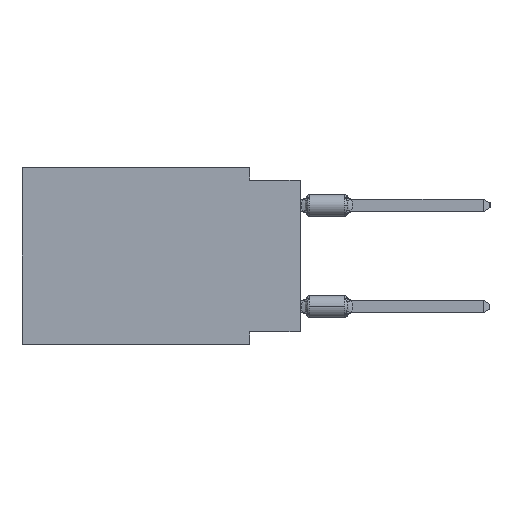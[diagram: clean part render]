
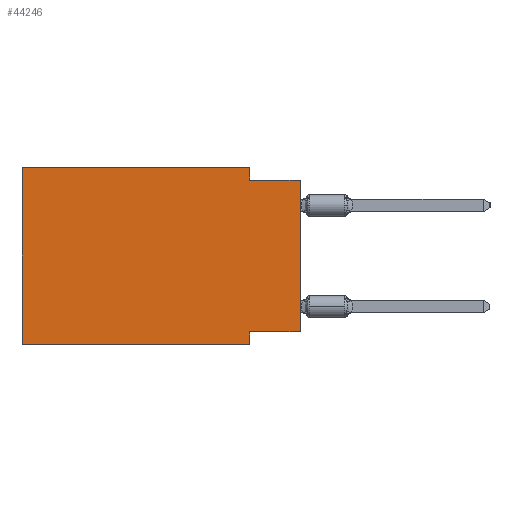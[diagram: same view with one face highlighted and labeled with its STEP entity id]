
A CAD part, left-side view. The second image highlights one B-rep face of the part: STEP entity #44246.
In plain terms, the highlighted planar face has unit normal (-1, 0, 0).
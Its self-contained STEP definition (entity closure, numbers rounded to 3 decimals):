
#1835 = ORIENTED_EDGE ( 'NONE', *, *, #51182, .T. ) ;
#3428 = CARTESIAN_POINT ( 'NONE',  ( 0., 13.97, -8.89 ) ) ;
#3501 = CARTESIAN_POINT ( 'NONE',  ( 0., 0., 0. ) ) ;
#4410 = EDGE_LOOP ( 'NONE', ( #1835, #31331, #40558, #20042, #10663, #21115, #50394, #46017 ) ) ;
#5445 = CARTESIAN_POINT ( 'NONE',  ( 0., 2.54, -8.89 ) ) ;
#5760 = LINE ( 'NONE', #50559, #7010 ) ;
#6490 = LINE ( 'NONE', #42623, #39428 ) ;
#6607 = CARTESIAN_POINT ( 'NONE',  ( 0., 0., -0.635 ) ) ;
#7010 = VECTOR ( 'NONE', #9966, 1000. ) ;
#7203 = EDGE_CURVE ( 'NONE', #24662, #46092, #7670, .T. ) ;
#7670 = LINE ( 'NONE', #35640, #49870 ) ;
#8952 = VECTOR ( 'NONE', #48303, 1000. ) ;
#8970 = EDGE_CURVE ( 'NONE', #22387, #45088, #16314, .T. ) ;
#9172 = DIRECTION ( 'NONE',  ( 0., 0., 1. ) ) ;
#9966 = DIRECTION ( 'NONE',  ( 0., -1., 0. ) ) ;
#10162 = CARTESIAN_POINT ( 'NONE',  ( 0., 2.54, 0. ) ) ;
#10324 = CARTESIAN_POINT ( 'NONE',  ( 0., 0., -8.255 ) ) ;
#10663 = ORIENTED_EDGE ( 'NONE', *, *, #8970, .F. ) ;
#11103 = DIRECTION ( 'NONE',  ( 0., -1., 0. ) ) ;
#11385 = DIRECTION ( 'NONE',  ( 0., 1., 0. ) ) ;
#12673 = EDGE_CURVE ( 'NONE', #46092, #26354, #12846, .T. ) ;
#12705 = CARTESIAN_POINT ( 'NONE',  ( 0., 13.97, 0. ) ) ;
#12846 = LINE ( 'NONE', #5445, #33324 ) ;
#16314 = LINE ( 'NONE', #37124, #21404 ) ;
#16546 = AXIS2_PLACEMENT_3D ( 'NONE', #12705, #28784, #44879 ) ;
#16802 = DIRECTION ( 'NONE',  ( 0., 0., -1. ) ) ;
#20042 = ORIENTED_EDGE ( 'NONE', *, *, #45274, .F. ) ;
#20633 = FACE_OUTER_BOUND ( 'NONE', #4410, .T. ) ;
#21009 = DIRECTION ( 'NONE',  ( 0., 0., -1. ) ) ;
#21115 = ORIENTED_EDGE ( 'NONE', *, *, #33896, .T. ) ;
#21404 = VECTOR ( 'NONE', #9172, 1000. ) ;
#21499 = CARTESIAN_POINT ( 'NONE',  ( 0., 2.54, -8.89 ) ) ;
#22387 = VERTEX_POINT ( 'NONE', #3428 ) ;
#23865 = CARTESIAN_POINT ( 'NONE',  ( 0., 2.54, -0.635 ) ) ;
#24662 = VERTEX_POINT ( 'NONE', #10324 ) ;
#26354 = VERTEX_POINT ( 'NONE', #21499 ) ;
#28277 = LINE ( 'NONE', #3501, #8952 ) ;
#28784 = DIRECTION ( 'NONE',  ( 1., 0., 0. ) ) ;
#29190 = CARTESIAN_POINT ( 'NONE',  ( 0., 13.97, 0. ) ) ;
#29744 = VECTOR ( 'NONE', #11103, 1000. ) ;
#30632 = CARTESIAN_POINT ( 'NONE',  ( 0., 0., -0.635 ) ) ;
#31331 = ORIENTED_EDGE ( 'NONE', *, *, #36528, .F. ) ;
#32148 = VERTEX_POINT ( 'NONE', #6607 ) ;
#32846 = EDGE_CURVE ( 'NONE', #51308, #42504, #45780, .T. ) ;
#33324 = VECTOR ( 'NONE', #16802, 1000. ) ;
#33896 = EDGE_CURVE ( 'NONE', #22387, #26354, #5760, .T. ) ;
#35461 = CARTESIAN_POINT ( 'NONE',  ( 0., 2.54, -8.255 ) ) ;
#35640 = CARTESIAN_POINT ( 'NONE',  ( 0., 0., -8.255 ) ) ;
#36528 = EDGE_CURVE ( 'NONE', #42504, #32148, #46973, .T. ) ;
#37124 = CARTESIAN_POINT ( 'NONE',  ( 0., 13.97, 0. ) ) ;
#39428 = VECTOR ( 'NONE', #43152, 1000. ) ;
#40558 = ORIENTED_EDGE ( 'NONE', *, *, #32846, .F. ) ;
#41958 = CARTESIAN_POINT ( 'NONE',  ( 0., 2.54, 0. ) ) ;
#42504 = VERTEX_POINT ( 'NONE', #23865 ) ;
#42623 = CARTESIAN_POINT ( 'NONE',  ( 0., 13.97, 0. ) ) ;
#43152 = DIRECTION ( 'NONE',  ( 0., -1., 0. ) ) ;
#44246 = ADVANCED_FACE ( 'NONE', ( #20633 ), #48817, .F. ) ;
#44879 = DIRECTION ( 'NONE',  ( 0., 0., -1. ) ) ;
#45088 = VERTEX_POINT ( 'NONE', #29190 ) ;
#45274 = EDGE_CURVE ( 'NONE', #45088, #51308, #6490, .T. ) ;
#45780 = LINE ( 'NONE', #10162, #49862 ) ;
#46017 = ORIENTED_EDGE ( 'NONE', *, *, #7203, .F. ) ;
#46092 = VERTEX_POINT ( 'NONE', #35461 ) ;
#46973 = LINE ( 'NONE', #30632, #29744 ) ;
#48303 = DIRECTION ( 'NONE',  ( 0., 0., 1. ) ) ;
#48817 = PLANE ( 'NONE',  #16546 ) ;
#49862 = VECTOR ( 'NONE', #21009, 1000. ) ;
#49870 = VECTOR ( 'NONE', #11385, 1000. ) ;
#50394 = ORIENTED_EDGE ( 'NONE', *, *, #12673, .F. ) ;
#50559 = CARTESIAN_POINT ( 'NONE',  ( 0., 13.97, -8.89 ) ) ;
#51182 = EDGE_CURVE ( 'NONE', #24662, #32148, #28277, .T. ) ;
#51308 = VERTEX_POINT ( 'NONE', #41958 ) ;
